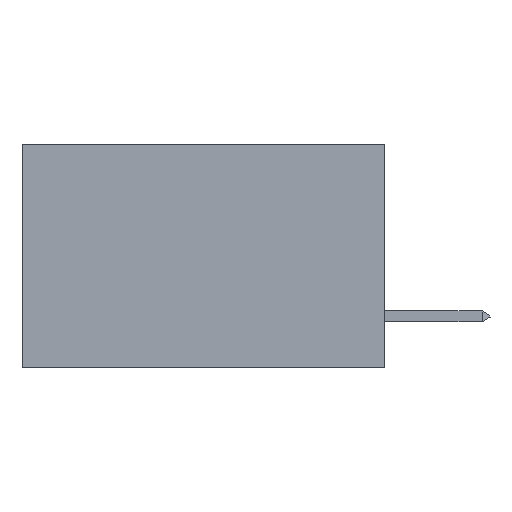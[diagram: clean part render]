
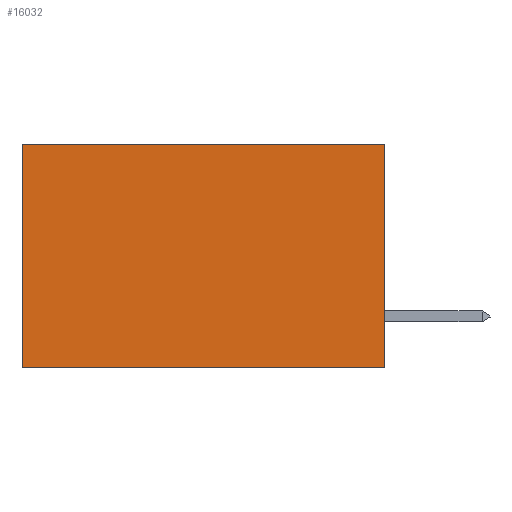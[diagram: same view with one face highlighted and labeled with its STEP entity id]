
A CAD part, left-side view. The second image highlights one B-rep face of the part: STEP entity #16032.
In plain terms, the highlighted planar face has unit normal (-1, 0, 0).
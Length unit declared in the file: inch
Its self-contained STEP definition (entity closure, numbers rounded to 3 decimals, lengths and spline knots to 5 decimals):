
#251 = CARTESIAN_POINT ( 'NONE',  ( 0.2875, 0., 0. ) ) ;
#372 = AXIS2_PLACEMENT_3D ( 'NONE', #18040, #15739, #18148 ) ;
#3216 = ORIENTED_EDGE ( 'NONE', *, *, #6451, .T. ) ;
#4148 = EDGE_CURVE ( 'NONE', #11201, #28007, #5638, .T. ) ;
#4733 = VERTEX_POINT ( 'NONE', #15459 ) ;
#5421 = LINE ( 'NONE', #13118, #21965 ) ;
#5638 = LINE ( 'NONE', #21871, #17011 ) ;
#6451 = EDGE_CURVE ( 'NONE', #4733, #11201, #10844, .T. ) ;
#8225 = CARTESIAN_POINT ( 'NONE',  ( 0.2875, 0., -0.37 ) ) ;
#8459 = VECTOR ( 'NONE', #27661, 39.37008 ) ;
#10844 = LINE ( 'NONE', #251, #8459 ) ;
#11201 = VERTEX_POINT ( 'NONE', #25910 ) ;
#11815 = EDGE_CURVE ( 'NONE', #18880, #28007, #27571, .T. ) ;
#13118 = CARTESIAN_POINT ( 'NONE',  ( 0.2875, 0., 0. ) ) ;
#15459 = CARTESIAN_POINT ( 'NONE',  ( 0.2875, 0., 0. ) ) ;
#15739 = DIRECTION ( 'NONE',  ( 1., 0., 0. ) ) ;
#16032 = ADVANCED_FACE ( 'NONE', ( #28440 ), #30422, .F. ) ;
#16447 = ORIENTED_EDGE ( 'NONE', *, *, #11815, .F. ) ;
#17011 = VECTOR ( 'NONE', #29816, 39.37008 ) ;
#17858 = ORIENTED_EDGE ( 'NONE', *, *, #4148, .T. ) ;
#18040 = CARTESIAN_POINT ( 'NONE',  ( 0.2875, 0., 0. ) ) ;
#18148 = DIRECTION ( 'NONE',  ( 0., 0., -1. ) ) ;
#18880 = VERTEX_POINT ( 'NONE', #8225 ) ;
#18977 = CARTESIAN_POINT ( 'NONE',  ( 0.2875, 0.6, -0.37 ) ) ;
#21871 = CARTESIAN_POINT ( 'NONE',  ( 0.2875, 0.6, 0. ) ) ;
#21965 = VECTOR ( 'NONE', #31297, 39.37008 ) ;
#22594 = ORIENTED_EDGE ( 'NONE', *, *, #32385, .F. ) ;
#23098 = CARTESIAN_POINT ( 'NONE',  ( 0.2875, 0., -0.37 ) ) ;
#25910 = CARTESIAN_POINT ( 'NONE',  ( 0.2875, 0.6, 0. ) ) ;
#27571 = LINE ( 'NONE', #23098, #28352 ) ;
#27661 = DIRECTION ( 'NONE',  ( 0., 1., 0. ) ) ;
#28007 = VERTEX_POINT ( 'NONE', #18977 ) ;
#28352 = VECTOR ( 'NONE', #30515, 39.37008 ) ;
#28440 = FACE_OUTER_BOUND ( 'NONE', #31323, .T. ) ;
#29816 = DIRECTION ( 'NONE',  ( 0., 0., -1. ) ) ;
#30422 = PLANE ( 'NONE',  #372 ) ;
#30515 = DIRECTION ( 'NONE',  ( 0., 1., 0. ) ) ;
#31297 = DIRECTION ( 'NONE',  ( 0., 0., -1. ) ) ;
#31323 = EDGE_LOOP ( 'NONE', ( #17858, #16447, #22594, #3216 ) ) ;
#32385 = EDGE_CURVE ( 'NONE', #4733, #18880, #5421, .T. ) ;
